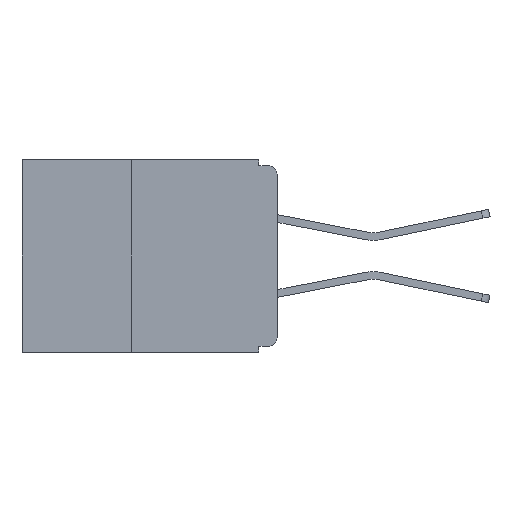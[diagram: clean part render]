
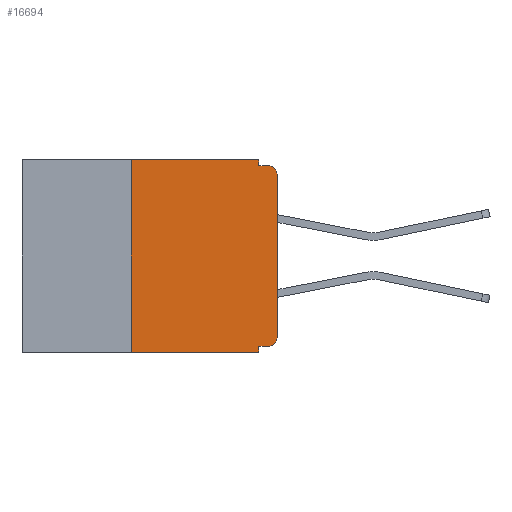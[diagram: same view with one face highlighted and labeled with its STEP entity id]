
A CAD part, left-side view. The second image highlights one B-rep face of the part: STEP entity #16694.
In plain terms, the highlighted planar face has unit normal (-1, 0, 0).
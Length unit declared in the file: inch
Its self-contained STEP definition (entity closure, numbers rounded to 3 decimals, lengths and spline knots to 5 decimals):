
#35 = CARTESIAN_POINT ( 'NONE',  ( 0., 0.031, -0.33 ) ) ;
#50 = ORIENTED_EDGE ( 'NONE', *, *, #21555, .T. ) ;
#285 = DIRECTION ( 'NONE',  ( 0., 0., -1. ) ) ;
#839 = AXIS2_PLACEMENT_3D ( 'NONE', #20962, #10784, #285 ) ;
#1379 = VECTOR ( 'NONE', #19547, 39.37008 ) ;
#1466 = CARTESIAN_POINT ( 'NONE',  ( 0., 0.015, -0.01 ) ) ;
#1566 = CARTESIAN_POINT ( 'NONE',  ( 0., 0.25, -0.33 ) ) ;
#1767 = DIRECTION ( 'NONE',  ( 0., 0., -1. ) ) ;
#1915 = ORIENTED_EDGE ( 'NONE', *, *, #3390, .F. ) ;
#1930 = LINE ( 'NONE', #3989, #1379 ) ;
#2240 = VERTEX_POINT ( 'NONE', #4775 ) ;
#2382 = CARTESIAN_POINT ( 'NONE',  ( 0., 0.015, -0.025 ) ) ;
#2708 = CARTESIAN_POINT ( 'NONE',  ( 0., 0.031, -0.32 ) ) ;
#2772 = ORIENTED_EDGE ( 'NONE', *, *, #9423, .T. ) ;
#2851 = ORIENTED_EDGE ( 'NONE', *, *, #11461, .F. ) ;
#3390 = EDGE_CURVE ( 'NONE', #5589, #10231, #12281, .T. ) ;
#3657 = CARTESIAN_POINT ( 'NONE',  ( 0., 0.031, 0. ) ) ;
#3873 = CIRCLE ( 'NONE', #839, 0.015 ) ;
#3989 = CARTESIAN_POINT ( 'NONE',  ( 0., 0., 0. ) ) ;
#4165 = DIRECTION ( 'NONE',  ( 0., 0., -1. ) ) ;
#4692 = VECTOR ( 'NONE', #12374, 39.37008 ) ;
#4775 = CARTESIAN_POINT ( 'NONE',  ( 0., 0., -0.025 ) ) ;
#4978 = EDGE_CURVE ( 'NONE', #10231, #16163, #16813, .T. ) ;
#5240 = LINE ( 'NONE', #35, #4692 ) ;
#5589 = VERTEX_POINT ( 'NONE', #20621 ) ;
#6209 = EDGE_CURVE ( 'NONE', #11877, #18084, #7810, .T. ) ;
#6465 = VERTEX_POINT ( 'NONE', #2708 ) ;
#6695 = EDGE_CURVE ( 'NONE', #12358, #6465, #9720, .T. ) ;
#6752 = AXIS2_PLACEMENT_3D ( 'NONE', #2382, #14622, #4165 ) ;
#7616 = CARTESIAN_POINT ( 'NONE',  ( 0., 0.031, -0.33 ) ) ;
#7633 = VECTOR ( 'NONE', #7645, 39.37008 ) ;
#7637 = VERTEX_POINT ( 'NONE', #7616 ) ;
#7645 = DIRECTION ( 'NONE',  ( 0., 0., 1. ) ) ;
#7810 = LINE ( 'NONE', #9080, #19903 ) ;
#8643 = DIRECTION ( 'NONE',  ( 0., 1., 0. ) ) ;
#8686 = LINE ( 'NONE', #19991, #12234 ) ;
#8731 = DIRECTION ( 'NONE',  ( 0., 0., -1. ) ) ;
#8853 = DIRECTION ( 'NONE',  ( 0., -1., 0. ) ) ;
#8871 = CIRCLE ( 'NONE', #6752, 0.015 ) ;
#9080 = CARTESIAN_POINT ( 'NONE',  ( 0., 0., -0.01 ) ) ;
#9331 = CARTESIAN_POINT ( 'NONE',  ( 0., 0.015, -0.32 ) ) ;
#9423 = EDGE_CURVE ( 'NONE', #2240, #18084, #8871, .T. ) ;
#9720 = LINE ( 'NONE', #15552, #18315 ) ;
#9806 = VERTEX_POINT ( 'NONE', #19452 ) ;
#10231 = VERTEX_POINT ( 'NONE', #10291 ) ;
#10286 = AXIS2_PLACEMENT_3D ( 'NONE', #15677, #12291, #1767 ) ;
#10291 = CARTESIAN_POINT ( 'NONE',  ( 0., 0.25, 0. ) ) ;
#10784 = DIRECTION ( 'NONE',  ( -1., 0., 0. ) ) ;
#11036 = EDGE_CURVE ( 'NONE', #9806, #2240, #1930, .T. ) ;
#11353 = ORIENTED_EDGE ( 'NONE', *, *, #6209, .F. ) ;
#11461 = EDGE_CURVE ( 'NONE', #16163, #11877, #15843, .T. ) ;
#11862 = ORIENTED_EDGE ( 'NONE', *, *, #6695, .F. ) ;
#11877 = VERTEX_POINT ( 'NONE', #15022 ) ;
#11948 = CARTESIAN_POINT ( 'NONE',  ( 0., 0.437, 0. ) ) ;
#12234 = VECTOR ( 'NONE', #18317, 39.37008 ) ;
#12241 = VECTOR ( 'NONE', #18797, 39.37008 ) ;
#12281 = LINE ( 'NONE', #1566, #7633 ) ;
#12291 = DIRECTION ( 'NONE',  ( 1., 0., 0. ) ) ;
#12358 = VERTEX_POINT ( 'NONE', #9331 ) ;
#12374 = DIRECTION ( 'NONE',  ( 0., 0., -1. ) ) ;
#12961 = ORIENTED_EDGE ( 'NONE', *, *, #22154, .F. ) ;
#13156 = ORIENTED_EDGE ( 'NONE', *, *, #13670, .T. ) ;
#13670 = EDGE_CURVE ( 'NONE', #5589, #7637, #8686, .T. ) ;
#14622 = DIRECTION ( 'NONE',  ( -1., 0., 0. ) ) ;
#15022 = CARTESIAN_POINT ( 'NONE',  ( 0., 0.031, -0.01 ) ) ;
#15321 = FACE_OUTER_BOUND ( 'NONE', #17875, .T. ) ;
#15552 = CARTESIAN_POINT ( 'NONE',  ( 0., 0., -0.32 ) ) ;
#15677 = CARTESIAN_POINT ( 'NONE',  ( 0., 0.437, 0. ) ) ;
#15843 = LINE ( 'NONE', #20679, #20817 ) ;
#16163 = VERTEX_POINT ( 'NONE', #3657 ) ;
#16694 = ADVANCED_FACE ( 'NONE', ( #15321 ), #20728, .F. ) ;
#16813 = LINE ( 'NONE', #11948, #12241 ) ;
#17875 = EDGE_LOOP ( 'NONE', ( #18542, #2772, #11353, #2851, #20256, #1915, #13156, #12961, #11862, #50 ) ) ;
#18084 = VERTEX_POINT ( 'NONE', #1466 ) ;
#18315 = VECTOR ( 'NONE', #8643, 39.37008 ) ;
#18317 = DIRECTION ( 'NONE',  ( 0., -1., 0. ) ) ;
#18542 = ORIENTED_EDGE ( 'NONE', *, *, #11036, .T. ) ;
#18797 = DIRECTION ( 'NONE',  ( 0., -1., 0. ) ) ;
#19452 = CARTESIAN_POINT ( 'NONE',  ( 0., 0., -0.305 ) ) ;
#19547 = DIRECTION ( 'NONE',  ( 0., 0., 1. ) ) ;
#19903 = VECTOR ( 'NONE', #8853, 39.37008 ) ;
#19991 = CARTESIAN_POINT ( 'NONE',  ( 0., 0.437, -0.33 ) ) ;
#20256 = ORIENTED_EDGE ( 'NONE', *, *, #4978, .F. ) ;
#20621 = CARTESIAN_POINT ( 'NONE',  ( 0., 0.25, -0.33 ) ) ;
#20679 = CARTESIAN_POINT ( 'NONE',  ( 0., 0.031, 0. ) ) ;
#20728 = PLANE ( 'NONE',  #10286 ) ;
#20817 = VECTOR ( 'NONE', #8731, 39.37008 ) ;
#20962 = CARTESIAN_POINT ( 'NONE',  ( 0., 0.015, -0.305 ) ) ;
#21555 = EDGE_CURVE ( 'NONE', #12358, #9806, #3873, .T. ) ;
#22154 = EDGE_CURVE ( 'NONE', #6465, #7637, #5240, .T. ) ;
